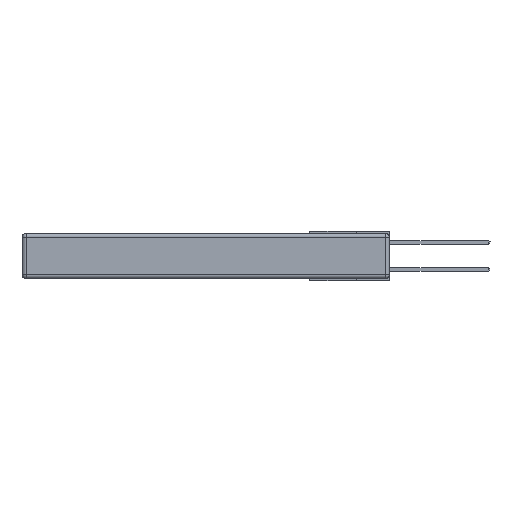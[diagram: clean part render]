
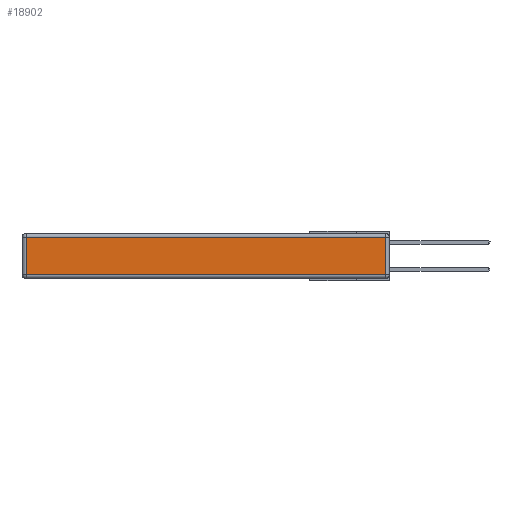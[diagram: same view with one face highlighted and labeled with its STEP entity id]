
A CAD part, left-side view. The second image highlights one B-rep face of the part: STEP entity #18902.
In plain terms, the highlighted planar face has unit normal (-1, 0, 0).
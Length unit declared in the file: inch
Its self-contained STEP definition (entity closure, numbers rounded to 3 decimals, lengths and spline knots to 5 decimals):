
#93 = VECTOR ( 'NONE', #2213, 39.37008 ) ;
#378 = LINE ( 'NONE', #21240, #93 ) ;
#2024 = CARTESIAN_POINT ( 'NONE',  ( 0., 2.72, -0.313 ) ) ;
#2213 = DIRECTION ( 'NONE',  ( 0., -1., 0. ) ) ;
#2473 = CARTESIAN_POINT ( 'NONE',  ( 0., 2.72, -0.343 ) ) ;
#2494 = LINE ( 'NONE', #20969, #11144 ) ;
#2499 = CARTESIAN_POINT ( 'NONE',  ( 0., 0.03, -0.313 ) ) ;
#3175 = VERTEX_POINT ( 'NONE', #2024 ) ;
#4597 = EDGE_CURVE ( 'NONE', #10299, #8927, #12944, .T. ) ;
#5096 = CARTESIAN_POINT ( 'NONE',  ( 0., 0.03, -0.343 ) ) ;
#5106 = VECTOR ( 'NONE', #15326, 39.37008 ) ;
#6065 = CARTESIAN_POINT ( 'NONE',  ( 0., 2.72, -0.03 ) ) ;
#8406 = LINE ( 'NONE', #2473, #8686 ) ;
#8686 = VECTOR ( 'NONE', #16439, 39.37008 ) ;
#8819 = ORIENTED_EDGE ( 'NONE', *, *, #14915, .T. ) ;
#8927 = VERTEX_POINT ( 'NONE', #13283 ) ;
#9372 = FACE_OUTER_BOUND ( 'NONE', #15149, .T. ) ;
#9373 = EDGE_CURVE ( 'NONE', #20976, #3175, #8406, .T. ) ;
#10299 = VERTEX_POINT ( 'NONE', #2499 ) ;
#10491 = DIRECTION ( 'NONE',  ( 0., 1., 0. ) ) ;
#11144 = VECTOR ( 'NONE', #10491, 39.37008 ) ;
#11395 = DIRECTION ( 'NONE',  ( 0., 0., 1. ) ) ;
#12072 = ORIENTED_EDGE ( 'NONE', *, *, #21115, .T. ) ;
#12944 = LINE ( 'NONE', #5096, #5106 ) ;
#13072 = CARTESIAN_POINT ( 'NONE',  ( 0., 0., -0.343 ) ) ;
#13283 = CARTESIAN_POINT ( 'NONE',  ( 0., 0.03, -0.03 ) ) ;
#14915 = EDGE_CURVE ( 'NONE', #3175, #10299, #378, .T. ) ;
#14920 = DIRECTION ( 'NONE',  ( -1., 0., 0. ) ) ;
#15024 = AXIS2_PLACEMENT_3D ( 'NONE', #13072, #14920, #11395 ) ;
#15149 = EDGE_LOOP ( 'NONE', ( #8819, #17153, #12072, #20462 ) ) ;
#15326 = DIRECTION ( 'NONE',  ( 0., 0., 1. ) ) ;
#16439 = DIRECTION ( 'NONE',  ( 0., 0., -1. ) ) ;
#17153 = ORIENTED_EDGE ( 'NONE', *, *, #4597, .T. ) ;
#18902 = ADVANCED_FACE ( 'NONE', ( #9372 ), #20361, .T. ) ;
#20361 = PLANE ( 'NONE',  #15024 ) ;
#20462 = ORIENTED_EDGE ( 'NONE', *, *, #9373, .T. ) ;
#20969 = CARTESIAN_POINT ( 'NONE',  ( 0., 2.75, -0.03 ) ) ;
#20976 = VERTEX_POINT ( 'NONE', #6065 ) ;
#21115 = EDGE_CURVE ( 'NONE', #8927, #20976, #2494, .T. ) ;
#21240 = CARTESIAN_POINT ( 'NONE',  ( 0., 0., -0.313 ) ) ;
